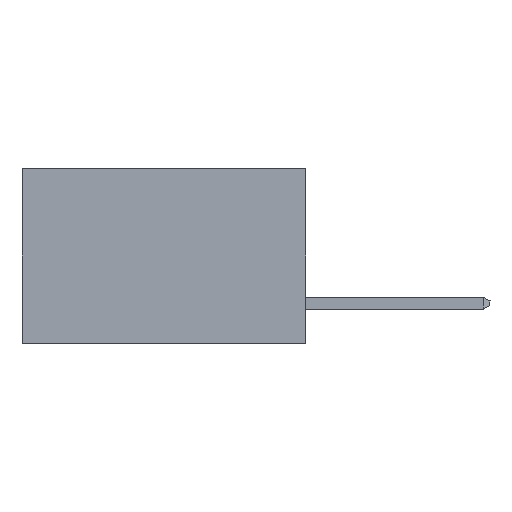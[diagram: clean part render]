
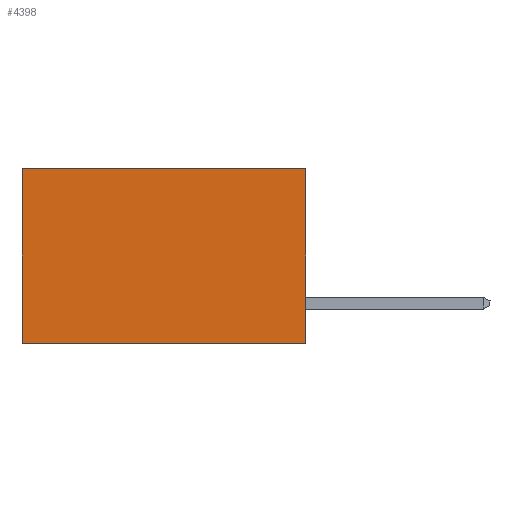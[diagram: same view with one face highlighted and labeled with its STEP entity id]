
A CAD part, left-side view. The second image highlights one B-rep face of the part: STEP entity #4398.
In plain terms, the highlighted planar face has unit normal (-1, 0, 0).
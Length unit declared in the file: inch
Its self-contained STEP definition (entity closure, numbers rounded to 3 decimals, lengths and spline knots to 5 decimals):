
#7 = LINE ( 'NONE', #13757, #8007 ) ;
#76 = DIRECTION ( 'NONE',  ( 0., 1., 0. ) ) ;
#571 = EDGE_CURVE ( 'NONE', #4128, #1451, #2253, .T. ) ;
#796 = CARTESIAN_POINT ( 'NONE',  ( 0.298, 0., 0. ) ) ;
#1451 = VERTEX_POINT ( 'NONE', #4750 ) ;
#1679 = ORIENTED_EDGE ( 'NONE', *, *, #17131, .F. ) ;
#1922 = VERTEX_POINT ( 'NONE', #6729 ) ;
#2253 = LINE ( 'NONE', #2733, #15274 ) ;
#2733 = CARTESIAN_POINT ( 'NONE',  ( 0.298, 0., -0.37 ) ) ;
#3053 = DIRECTION ( 'NONE',  ( 0., 0., -1. ) ) ;
#4128 = VERTEX_POINT ( 'NONE', #14494 ) ;
#4398 = ADVANCED_FACE ( 'NONE', ( #17036 ), #16914, .F. ) ;
#4750 = CARTESIAN_POINT ( 'NONE',  ( 0.298, 0.6, -0.37 ) ) ;
#4815 = DIRECTION ( 'NONE',  ( 0., 0., -1. ) ) ;
#4936 = DIRECTION ( 'NONE',  ( 0., 0., -1. ) ) ;
#5287 = LINE ( 'NONE', #10812, #7213 ) ;
#5385 = EDGE_LOOP ( 'NONE', ( #15244, #16437, #1679, #15002 ) ) ;
#6729 = CARTESIAN_POINT ( 'NONE',  ( 0.298, 0., 0. ) ) ;
#7213 = VECTOR ( 'NONE', #16367, 39.37008 ) ;
#7407 = CARTESIAN_POINT ( 'NONE',  ( 0.298, 0.6, 0. ) ) ;
#7490 = CARTESIAN_POINT ( 'NONE',  ( 0.298, 0.6, 0. ) ) ;
#8007 = VECTOR ( 'NONE', #3053, 39.37008 ) ;
#9137 = VECTOR ( 'NONE', #4936, 39.37008 ) ;
#9865 = EDGE_CURVE ( 'NONE', #12501, #1451, #15831, .T. ) ;
#9894 = EDGE_CURVE ( 'NONE', #1922, #12501, #5287, .T. ) ;
#10812 = CARTESIAN_POINT ( 'NONE',  ( 0.298, 0., 0. ) ) ;
#12501 = VERTEX_POINT ( 'NONE', #7407 ) ;
#13057 = DIRECTION ( 'NONE',  ( 1., 0., 0. ) ) ;
#13230 = AXIS2_PLACEMENT_3D ( 'NONE', #796, #13057, #4815 ) ;
#13757 = CARTESIAN_POINT ( 'NONE',  ( 0.298, 0., 0. ) ) ;
#14494 = CARTESIAN_POINT ( 'NONE',  ( 0.298, 0., -0.37 ) ) ;
#15002 = ORIENTED_EDGE ( 'NONE', *, *, #9894, .T. ) ;
#15244 = ORIENTED_EDGE ( 'NONE', *, *, #9865, .T. ) ;
#15274 = VECTOR ( 'NONE', #76, 39.37008 ) ;
#15831 = LINE ( 'NONE', #7490, #9137 ) ;
#16367 = DIRECTION ( 'NONE',  ( 0., 1., 0. ) ) ;
#16437 = ORIENTED_EDGE ( 'NONE', *, *, #571, .F. ) ;
#16914 = PLANE ( 'NONE',  #13230 ) ;
#17036 = FACE_OUTER_BOUND ( 'NONE', #5385, .T. ) ;
#17131 = EDGE_CURVE ( 'NONE', #1922, #4128, #7, .T. ) ;
